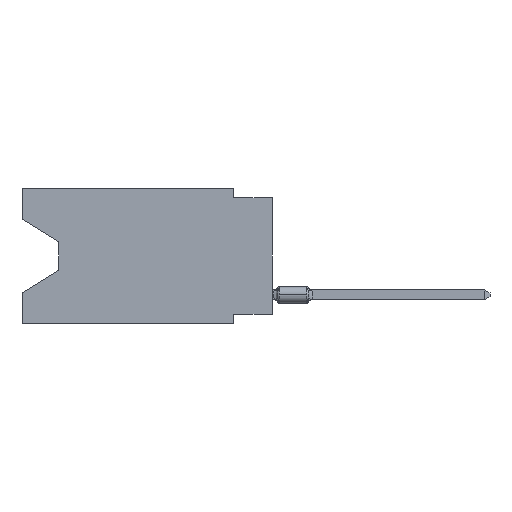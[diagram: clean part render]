
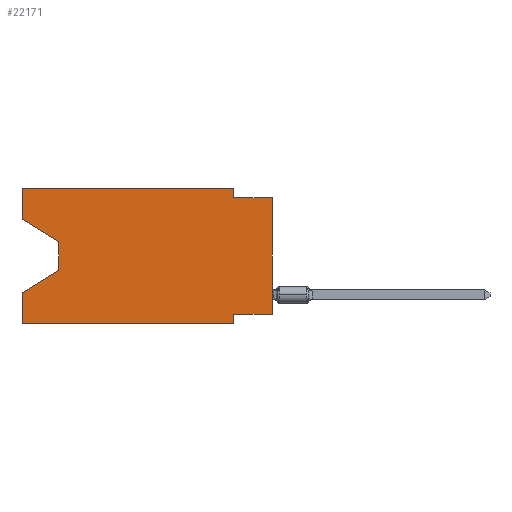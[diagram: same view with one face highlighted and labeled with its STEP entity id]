
A CAD part, left-side view. The second image highlights one B-rep face of the part: STEP entity #22171.
In plain terms, the highlighted planar face has unit normal (-1, 0, 0).
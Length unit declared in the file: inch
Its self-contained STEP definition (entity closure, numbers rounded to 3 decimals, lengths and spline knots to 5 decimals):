
#356 = ORIENTED_EDGE ( 'NONE', *, *, #19523, .F. ) ;
#360 = EDGE_LOOP ( 'NONE', ( #4615, #21035, #18785, #3480, #24496, #356, #6623, #11018, #13413, #984, #24166, #7889 ) ) ;
#782 = CARTESIAN_POINT ( 'NONE',  ( 0., 0.55, -0.212 ) ) ;
#901 = CARTESIAN_POINT ( 'NONE',  ( 0., 0.645, -0.08025 ) ) ;
#944 = CARTESIAN_POINT ( 'NONE',  ( 0., 0.1, -0.325 ) ) ;
#984 = ORIENTED_EDGE ( 'NONE', *, *, #22873, .F. ) ;
#1989 = CARTESIAN_POINT ( 'NONE',  ( 0., 0.55, -0.212 ) ) ;
#2268 = VERTEX_POINT ( 'NONE', #8730 ) ;
#2915 = DIRECTION ( 'NONE',  ( 0., 0., -1. ) ) ;
#3480 = ORIENTED_EDGE ( 'NONE', *, *, #20851, .F. ) ;
#3546 = CARTESIAN_POINT ( 'NONE',  ( 0., 0., 0. ) ) ;
#3704 = VECTOR ( 'NONE', #6614, 39.37008 ) ;
#3851 = CARTESIAN_POINT ( 'NONE',  ( 0., 0.645, 0. ) ) ;
#3888 = CARTESIAN_POINT ( 'NONE',  ( 0., 0.1, -0.025 ) ) ;
#4005 = CARTESIAN_POINT ( 'NONE',  ( 0., 0.55, -0.138 ) ) ;
#4140 = CARTESIAN_POINT ( 'NONE',  ( 0., 0.645, 0. ) ) ;
#4417 = EDGE_CURVE ( 'NONE', #15283, #9568, #25393, .T. ) ;
#4549 = EDGE_CURVE ( 'NONE', #19732, #22929, #11941, .T. ) ;
#4586 = DIRECTION ( 'NONE',  ( 0., -1., 0. ) ) ;
#4615 = ORIENTED_EDGE ( 'NONE', *, *, #4417, .T. ) ;
#5255 = DIRECTION ( 'NONE',  ( 0., -0.855, -0.519 ) ) ;
#5550 = VECTOR ( 'NONE', #15662, 39.37008 ) ;
#5636 = DIRECTION ( 'NONE',  ( 0., -1., 0. ) ) ;
#6135 = EDGE_CURVE ( 'NONE', #14757, #2268, #7862, .T. ) ;
#6478 = VECTOR ( 'NONE', #4586, 39.37008 ) ;
#6614 = DIRECTION ( 'NONE',  ( 0., 0., -1. ) ) ;
#6623 = ORIENTED_EDGE ( 'NONE', *, *, #14471, .F. ) ;
#7150 = VECTOR ( 'NONE', #21148, 39.37008 ) ;
#7533 = LINE ( 'NONE', #4005, #22691 ) ;
#7800 = VERTEX_POINT ( 'NONE', #4140 ) ;
#7862 = LINE ( 'NONE', #3546, #12094 ) ;
#7889 = ORIENTED_EDGE ( 'NONE', *, *, #20329, .F. ) ;
#8138 = DIRECTION ( 'NONE',  ( 0., 0.855, -0.519 ) ) ;
#8730 = CARTESIAN_POINT ( 'NONE',  ( 0., 0., -0.025 ) ) ;
#8805 = VECTOR ( 'NONE', #19255, 39.37008 ) ;
#9568 = VERTEX_POINT ( 'NONE', #24458 ) ;
#9999 = CARTESIAN_POINT ( 'NONE',  ( 0., 0., -0.325 ) ) ;
#11018 = ORIENTED_EDGE ( 'NONE', *, *, #6135, .T. ) ;
#11252 = CARTESIAN_POINT ( 'NONE',  ( 0., 0.1, -0.35 ) ) ;
#11294 = LINE ( 'NONE', #21604, #8805 ) ;
#11803 = DIRECTION ( 'NONE',  ( 0., 0., 1. ) ) ;
#11941 = LINE ( 'NONE', #1989, #21069 ) ;
#12094 = VECTOR ( 'NONE', #11803, 39.37008 ) ;
#12254 = AXIS2_PLACEMENT_3D ( 'NONE', #20336, #14691, #2915 ) ;
#12656 = LINE ( 'NONE', #18924, #21922 ) ;
#13413 = ORIENTED_EDGE ( 'NONE', *, *, #16441, .F. ) ;
#13612 = VERTEX_POINT ( 'NONE', #944 ) ;
#13648 = VERTEX_POINT ( 'NONE', #19396 ) ;
#14198 = DIRECTION ( 'NONE',  ( 0., 0., 1. ) ) ;
#14471 = EDGE_CURVE ( 'NONE', #14757, #13612, #17365, .T. ) ;
#14566 = FACE_OUTER_BOUND ( 'NONE', #360, .T. ) ;
#14691 = DIRECTION ( 'NONE',  ( 1., 0., 0. ) ) ;
#14757 = VERTEX_POINT ( 'NONE', #9999 ) ;
#15227 = VECTOR ( 'NONE', #5255, 39.37008 ) ;
#15283 = VERTEX_POINT ( 'NONE', #901 ) ;
#15429 = EDGE_CURVE ( 'NONE', #9568, #19732, #7533, .T. ) ;
#15662 = DIRECTION ( 'NONE',  ( 0., 1., 0. ) ) ;
#16164 = LINE ( 'NONE', #3851, #17619 ) ;
#16441 = EDGE_CURVE ( 'NONE', #22749, #2268, #19084, .T. ) ;
#16606 = VERTEX_POINT ( 'NONE', #11252 ) ;
#17365 = LINE ( 'NONE', #23242, #5550 ) ;
#17433 = VERTEX_POINT ( 'NONE', #25794 ) ;
#17619 = VECTOR ( 'NONE', #14198, 39.37008 ) ;
#18091 = EDGE_CURVE ( 'NONE', #17433, #16606, #12656, .T. ) ;
#18785 = ORIENTED_EDGE ( 'NONE', *, *, #4549, .T. ) ;
#18924 = CARTESIAN_POINT ( 'NONE',  ( 0., 0.645, -0.35 ) ) ;
#19084 = LINE ( 'NONE', #20670, #6478 ) ;
#19255 = DIRECTION ( 'NONE',  ( 0., 0., -1. ) ) ;
#19396 = CARTESIAN_POINT ( 'NONE',  ( 0., 0.1, 0. ) ) ;
#19523 = EDGE_CURVE ( 'NONE', #13612, #16606, #11294, .T. ) ;
#19528 = CARTESIAN_POINT ( 'NONE',  ( 0., 0.645, -0.26975 ) ) ;
#19732 = VERTEX_POINT ( 'NONE', #782 ) ;
#20329 = EDGE_CURVE ( 'NONE', #15283, #7800, #25598, .T. ) ;
#20336 = CARTESIAN_POINT ( 'NONE',  ( 0., 0.645, 0. ) ) ;
#20510 = DIRECTION ( 'NONE',  ( 0., -1., 0. ) ) ;
#20670 = CARTESIAN_POINT ( 'NONE',  ( 0., 0., -0.025 ) ) ;
#20851 = EDGE_CURVE ( 'NONE', #17433, #22929, #16164, .T. ) ;
#21035 = ORIENTED_EDGE ( 'NONE', *, *, #15429, .T. ) ;
#21069 = VECTOR ( 'NONE', #8138, 39.37008 ) ;
#21148 = DIRECTION ( 'NONE',  ( 0., 0., 1. ) ) ;
#21455 = CARTESIAN_POINT ( 'NONE',  ( 0., 0.645, 0. ) ) ;
#21604 = CARTESIAN_POINT ( 'NONE',  ( 0., 0.1, -0.35 ) ) ;
#21922 = VECTOR ( 'NONE', #20510, 39.37008 ) ;
#22171 = ADVANCED_FACE ( 'NONE', ( #14566 ), #24759, .F. ) ;
#22691 = VECTOR ( 'NONE', #25846, 39.37008 ) ;
#22749 = VERTEX_POINT ( 'NONE', #3888 ) ;
#22822 = LINE ( 'NONE', #24536, #3704 ) ;
#22873 = EDGE_CURVE ( 'NONE', #13648, #22749, #22822, .T. ) ;
#22929 = VERTEX_POINT ( 'NONE', #19528 ) ;
#23171 = CARTESIAN_POINT ( 'NONE',  ( 0., 0.645, -0.08025 ) ) ;
#23242 = CARTESIAN_POINT ( 'NONE',  ( 0., 0., -0.325 ) ) ;
#23296 = EDGE_CURVE ( 'NONE', #7800, #13648, #25778, .T. ) ;
#23362 = CARTESIAN_POINT ( 'NONE',  ( 0., 0.645, 0. ) ) ;
#24166 = ORIENTED_EDGE ( 'NONE', *, *, #23296, .F. ) ;
#24458 = CARTESIAN_POINT ( 'NONE',  ( 0., 0.55, -0.138 ) ) ;
#24496 = ORIENTED_EDGE ( 'NONE', *, *, #18091, .T. ) ;
#24536 = CARTESIAN_POINT ( 'NONE',  ( 0., 0.1, 0. ) ) ;
#24759 = PLANE ( 'NONE',  #12254 ) ;
#25393 = LINE ( 'NONE', #23171, #15227 ) ;
#25462 = VECTOR ( 'NONE', #5636, 39.37008 ) ;
#25598 = LINE ( 'NONE', #23362, #7150 ) ;
#25778 = LINE ( 'NONE', #21455, #25462 ) ;
#25794 = CARTESIAN_POINT ( 'NONE',  ( 0., 0.645, -0.35 ) ) ;
#25846 = DIRECTION ( 'NONE',  ( 0., 0., -1. ) ) ;
